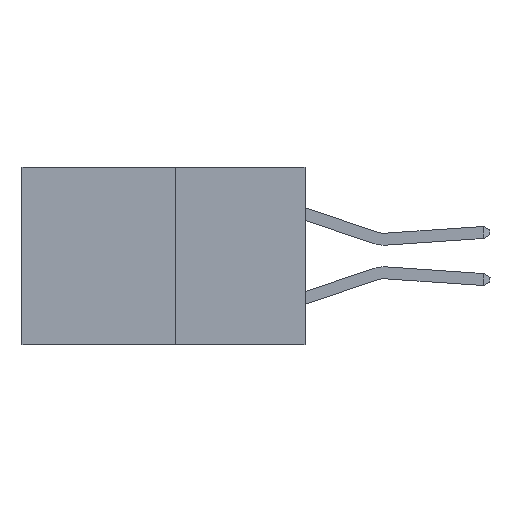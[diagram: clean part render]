
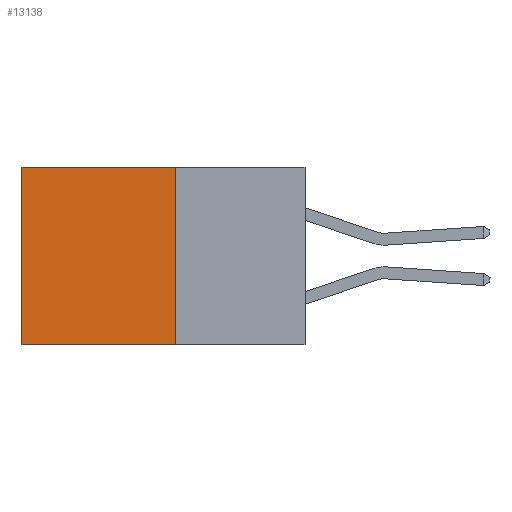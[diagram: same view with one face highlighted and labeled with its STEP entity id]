
A CAD part, left-side view. The second image highlights one B-rep face of the part: STEP entity #13138.
In plain terms, the highlighted planar face has unit normal (-1, 0, 0).
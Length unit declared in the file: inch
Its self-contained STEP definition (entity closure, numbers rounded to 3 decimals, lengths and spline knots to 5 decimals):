
#766 = VERTEX_POINT ( 'NONE', #17727 ) ;
#1614 = VECTOR ( 'NONE', #11628, 39.37008 ) ;
#2517 = LINE ( 'NONE', #18316, #6532 ) ;
#3802 = CARTESIAN_POINT ( 'NONE',  ( 0.277, 0.59, 0. ) ) ;
#4219 = CARTESIAN_POINT ( 'NONE',  ( 0.277, 0.27, 0. ) ) ;
#4444 = CARTESIAN_POINT ( 'NONE',  ( 0.277, 0.59, -0.37 ) ) ;
#6079 = DIRECTION ( 'NONE',  ( 0., 1., 0. ) ) ;
#6532 = VECTOR ( 'NONE', #11323, 39.37008 ) ;
#6734 = EDGE_CURVE ( 'NONE', #7207, #18446, #15116, .T. ) ;
#6887 = LINE ( 'NONE', #14573, #13958 ) ;
#7207 = VERTEX_POINT ( 'NONE', #3802 ) ;
#7488 = VERTEX_POINT ( 'NONE', #4219 ) ;
#7588 = VECTOR ( 'NONE', #10493, 39.37008 ) ;
#7628 = EDGE_CURVE ( 'NONE', #7488, #7207, #6887, .T. ) ;
#8053 = EDGE_LOOP ( 'NONE', ( #11550, #16186, #12713, #17092 ) ) ;
#8763 = DIRECTION ( 'NONE',  ( 1., 0., 0. ) ) ;
#9660 = CARTESIAN_POINT ( 'NONE',  ( 0.277, 0.59, -0.37 ) ) ;
#10493 = DIRECTION ( 'NONE',  ( 0., 0., -1. ) ) ;
#11323 = DIRECTION ( 'NONE',  ( 0., 0., -1. ) ) ;
#11550 = ORIENTED_EDGE ( 'NONE', *, *, #6734, .T. ) ;
#11628 = DIRECTION ( 'NONE',  ( 0., 1., 0. ) ) ;
#11794 = EDGE_CURVE ( 'NONE', #766, #18446, #16575, .T. ) ;
#12713 = ORIENTED_EDGE ( 'NONE', *, *, #17980, .F. ) ;
#12968 = PLANE ( 'NONE',  #15147 ) ;
#13138 = ADVANCED_FACE ( 'NONE', ( #13244 ), #12968, .F. ) ;
#13244 = FACE_OUTER_BOUND ( 'NONE', #8053, .T. ) ;
#13958 = VECTOR ( 'NONE', #6079, 39.37008 ) ;
#14573 = CARTESIAN_POINT ( 'NONE',  ( 0.277, 0.27, 0. ) ) ;
#15116 = LINE ( 'NONE', #4444, #7588 ) ;
#15147 = AXIS2_PLACEMENT_3D ( 'NONE', #15819, #8763, #18569 ) ;
#15819 = CARTESIAN_POINT ( 'NONE',  ( 0.277, 0.27, -0.37 ) ) ;
#15917 = CARTESIAN_POINT ( 'NONE',  ( 0.277, 0.27, -0.37 ) ) ;
#16186 = ORIENTED_EDGE ( 'NONE', *, *, #11794, .F. ) ;
#16575 = LINE ( 'NONE', #15917, #1614 ) ;
#17092 = ORIENTED_EDGE ( 'NONE', *, *, #7628, .T. ) ;
#17727 = CARTESIAN_POINT ( 'NONE',  ( 0.277, 0.27, -0.37 ) ) ;
#17980 = EDGE_CURVE ( 'NONE', #7488, #766, #2517, .T. ) ;
#18316 = CARTESIAN_POINT ( 'NONE',  ( 0.277, 0.27, -0.37 ) ) ;
#18446 = VERTEX_POINT ( 'NONE', #9660 ) ;
#18569 = DIRECTION ( 'NONE',  ( 0., 0., -1. ) ) ;
